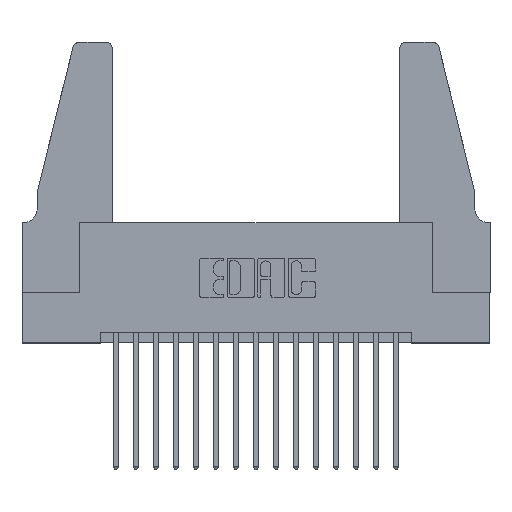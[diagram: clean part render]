
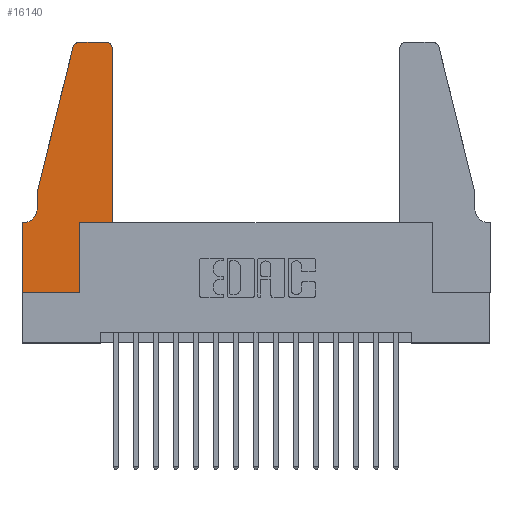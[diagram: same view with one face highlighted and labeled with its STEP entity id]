
A CAD part, top view. The second image highlights one B-rep face of the part: STEP entity #16140.
In plain terms, the highlighted planar face has unit normal (0, 0, 1).
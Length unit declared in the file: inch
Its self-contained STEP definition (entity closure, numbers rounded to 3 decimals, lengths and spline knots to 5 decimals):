
#32 = CARTESIAN_POINT ( 'NONE',  ( 0.4505, 0.35, 0.37 ) ) ;
#272 = VERTEX_POINT ( 'NONE', #4557 ) ;
#467 = CARTESIAN_POINT ( 'NONE',  ( 0.0755, 0.42, 0.37 ) ) ;
#616 = VERTEX_POINT ( 'NONE', #7151 ) ;
#694 = CIRCLE ( 'NONE', #13740, 0.07 ) ;
#1041 = DIRECTION ( 'NONE',  ( 1., 0., 0. ) ) ;
#1096 = LINE ( 'NONE', #5051, #14286 ) ;
#1155 = AXIS2_PLACEMENT_3D ( 'NONE', #8631, #4627, #13976 ) ;
#1484 = CARTESIAN_POINT ( 'NONE',  ( 0.2865, 0., 0.37 ) ) ;
#1531 = AXIS2_PLACEMENT_3D ( 'NONE', #17211, #9334, #1041 ) ;
#1682 = VERTEX_POINT ( 'NONE', #12958 ) ;
#1788 = DIRECTION ( 'NONE',  ( 1., 0., 0. ) ) ;
#1860 = LINE ( 'NONE', #8153, #11924 ) ;
#1982 = VERTEX_POINT ( 'NONE', #17360 ) ;
#2089 = EDGE_CURVE ( 'NONE', #11422, #3327, #16740, .T. ) ;
#2106 = DIRECTION ( 'NONE',  ( -0.239, -0.971, 0. ) ) ;
#2315 = EDGE_CURVE ( 'NONE', #616, #272, #9952, .T. ) ;
#2530 = VECTOR ( 'NONE', #12859, 39.37008 ) ;
#2625 = LINE ( 'NONE', #32, #16513 ) ;
#2645 = VECTOR ( 'NONE', #9135, 39.37008 ) ;
#2713 = AXIS2_PLACEMENT_3D ( 'NONE', #13229, #5193, #14503 ) ;
#2764 = VERTEX_POINT ( 'NONE', #467 ) ;
#2768 = CARTESIAN_POINT ( 'NONE',  ( 0.0755, 0.35, 0.37 ) ) ;
#2788 = EDGE_CURVE ( 'NONE', #3327, #14884, #2625, .T. ) ;
#2980 = LINE ( 'NONE', #4798, #2530 ) ;
#3122 = PLANE ( 'NONE',  #1155 ) ;
#3325 = ORIENTED_EDGE ( 'NONE', *, *, #15129, .T. ) ;
#3327 = VERTEX_POINT ( 'NONE', #3653 ) ;
#3653 = CARTESIAN_POINT ( 'NONE',  ( 0.4505, 0.35, 0.37 ) ) ;
#3930 = DIRECTION ( 'NONE',  ( 0., 0., -1. ) ) ;
#4557 = CARTESIAN_POINT ( 'NONE',  ( 0.284, 1.25, 0.37 ) ) ;
#4627 = DIRECTION ( 'NONE',  ( 0., 0., 1. ) ) ;
#4798 = CARTESIAN_POINT ( 'NONE',  ( 0., 0., 0.37 ) ) ;
#4831 = ORIENTED_EDGE ( 'NONE', *, *, #5504, .T. ) ;
#5023 = CIRCLE ( 'NONE', #2713, 0.03 ) ;
#5051 = CARTESIAN_POINT ( 'NONE',  ( 0.2865, 0.35, 0.37 ) ) ;
#5193 = DIRECTION ( 'NONE',  ( 0., 0., 1. ) ) ;
#5504 = EDGE_CURVE ( 'NONE', #14884, #616, #6927, .T. ) ;
#5511 = VECTOR ( 'NONE', #1788, 39.37008 ) ;
#5992 = ORIENTED_EDGE ( 'NONE', *, *, #10277, .T. ) ;
#6078 = EDGE_CURVE ( 'NONE', #272, #14934, #5023, .T. ) ;
#6435 = FACE_OUTER_BOUND ( 'NONE', #17233, .T. ) ;
#6927 = CIRCLE ( 'NONE', #1531, 0.03 ) ;
#7151 = CARTESIAN_POINT ( 'NONE',  ( 0.4205, 1.25, 0.37 ) ) ;
#7605 = CARTESIAN_POINT ( 'NONE',  ( 0.0755, 0.5, 0.37 ) ) ;
#7905 = EDGE_CURVE ( 'NONE', #2764, #1682, #694, .T. ) ;
#8153 = CARTESIAN_POINT ( 'NONE',  ( 0.0755, 0.5, 0.37 ) ) ;
#8631 = CARTESIAN_POINT ( 'NONE',  ( 0., 0.35, 0.37 ) ) ;
#8720 = CARTESIAN_POINT ( 'NONE',  ( 0., 0., 0.37 ) ) ;
#9135 = DIRECTION ( 'NONE',  ( -1., 0., 0. ) ) ;
#9334 = DIRECTION ( 'NONE',  ( 0., 0., 1. ) ) ;
#9519 = DIRECTION ( 'NONE',  ( 0., -1., 0. ) ) ;
#9658 = ORIENTED_EDGE ( 'NONE', *, *, #7905, .T. ) ;
#9668 = VERTEX_POINT ( 'NONE', #15645 ) ;
#9706 = EDGE_CURVE ( 'NONE', #17331, #11422, #1096, .T. ) ;
#9717 = CARTESIAN_POINT ( 'NONE',  ( 0.4505, 1.22, 0.37 ) ) ;
#9952 = LINE ( 'NONE', #14981, #2645 ) ;
#10277 = EDGE_CURVE ( 'NONE', #1982, #17331, #16119, .T. ) ;
#10321 = VERTEX_POINT ( 'NONE', #15422 ) ;
#10489 = DIRECTION ( 'NONE',  ( 0., 1., 0. ) ) ;
#11182 = CARTESIAN_POINT ( 'NONE',  ( 0.2865, 0.35, 0.37 ) ) ;
#11210 = ORIENTED_EDGE ( 'NONE', *, *, #15429, .T. ) ;
#11237 = LINE ( 'NONE', #2768, #14681 ) ;
#11422 = VERTEX_POINT ( 'NONE', #11182 ) ;
#11924 = VECTOR ( 'NONE', #9519, 39.37008 ) ;
#12055 = CARTESIAN_POINT ( 'NONE',  ( 0.0055, 0.42, 0.37 ) ) ;
#12815 = ORIENTED_EDGE ( 'NONE', *, *, #2315, .T. ) ;
#12859 = DIRECTION ( 'NONE',  ( 0., -1., 0. ) ) ;
#12958 = CARTESIAN_POINT ( 'NONE',  ( 0.0055, 0.35, 0.37 ) ) ;
#13127 = DIRECTION ( 'NONE',  ( 1., 0., 0. ) ) ;
#13146 = VECTOR ( 'NONE', #2106, 39.37008 ) ;
#13229 = CARTESIAN_POINT ( 'NONE',  ( 0.284, 1.22, 0.37 ) ) ;
#13286 = VECTOR ( 'NONE', #13127, 39.37008 ) ;
#13370 = DIRECTION ( 'NONE',  ( -1., 0., 0. ) ) ;
#13580 = ORIENTED_EDGE ( 'NONE', *, *, #2788, .T. ) ;
#13740 = AXIS2_PLACEMENT_3D ( 'NONE', #12055, #3930, #13370 ) ;
#13976 = DIRECTION ( 'NONE',  ( 1., 0., 0. ) ) ;
#14076 = ORIENTED_EDGE ( 'NONE', *, *, #9706, .T. ) ;
#14286 = VECTOR ( 'NONE', #10489, 39.37008 ) ;
#14503 = DIRECTION ( 'NONE',  ( 1., 0., 0. ) ) ;
#14681 = VECTOR ( 'NONE', #16186, 39.37008 ) ;
#14884 = VERTEX_POINT ( 'NONE', #9717 ) ;
#14934 = VERTEX_POINT ( 'NONE', #15069 ) ;
#14981 = CARTESIAN_POINT ( 'NONE',  ( 0.2605, 1.25, 0.37 ) ) ;
#15069 = CARTESIAN_POINT ( 'NONE',  ( 0.25487, 1.22718, 0.37 ) ) ;
#15092 = CARTESIAN_POINT ( 'NONE',  ( 0.4505, 0.35, 0.37 ) ) ;
#15129 = EDGE_CURVE ( 'NONE', #10321, #1982, #2980, .T. ) ;
#15379 = ORIENTED_EDGE ( 'NONE', *, *, #2089, .T. ) ;
#15422 = CARTESIAN_POINT ( 'NONE',  ( 0., 0.35, 0.37 ) ) ;
#15429 = EDGE_CURVE ( 'NONE', #9668, #2764, #1860, .T. ) ;
#15442 = DIRECTION ( 'NONE',  ( 0., 1., 0. ) ) ;
#15645 = CARTESIAN_POINT ( 'NONE',  ( 0.0755, 0.5, 0.37 ) ) ;
#15732 = EDGE_CURVE ( 'NONE', #14934, #9668, #16600, .T. ) ;
#16119 = LINE ( 'NONE', #8720, #5511 ) ;
#16140 = ADVANCED_FACE ( 'NONE', ( #6435 ), #3122, .T. ) ;
#16186 = DIRECTION ( 'NONE',  ( -1., 0., 0. ) ) ;
#16206 = ORIENTED_EDGE ( 'NONE', *, *, #6078, .T. ) ;
#16277 = ORIENTED_EDGE ( 'NONE', *, *, #17270, .T. ) ;
#16513 = VECTOR ( 'NONE', #15442, 39.37008 ) ;
#16600 = LINE ( 'NONE', #7605, #13146 ) ;
#16740 = LINE ( 'NONE', #15092, #13286 ) ;
#17022 = ORIENTED_EDGE ( 'NONE', *, *, #15732, .T. ) ;
#17211 = CARTESIAN_POINT ( 'NONE',  ( 0.4205, 1.22, 0.37 ) ) ;
#17233 = EDGE_LOOP ( 'NONE', ( #12815, #16206, #17022, #11210, #9658, #16277, #3325, #5992, #14076, #15379, #13580, #4831 ) ) ;
#17270 = EDGE_CURVE ( 'NONE', #1682, #10321, #11237, .T. ) ;
#17331 = VERTEX_POINT ( 'NONE', #1484 ) ;
#17360 = CARTESIAN_POINT ( 'NONE',  ( 0., 0., 0.37 ) ) ;
